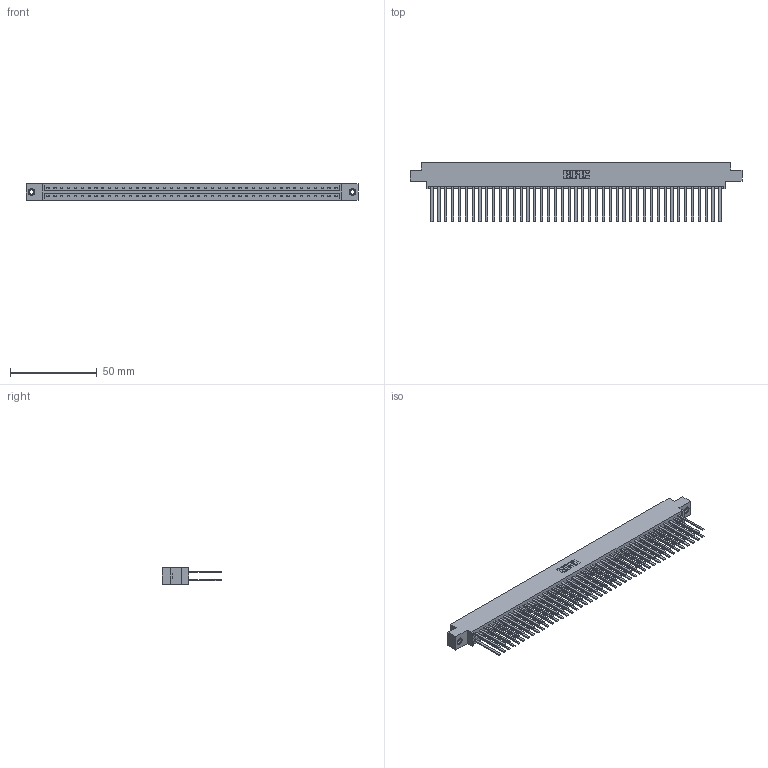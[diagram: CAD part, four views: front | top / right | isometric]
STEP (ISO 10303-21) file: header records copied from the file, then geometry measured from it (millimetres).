
FILE_DESCRIPTION (( 'STEP AP203' ), '1' );
FILE_NAME ('833-086-544-807.STEP', '2020-06-06T03:47:48', ( '' ), ( '' ), 'SwSTEP 2.0', 'SolidWorks 2020', '' );
FILE_SCHEMA (( 'CONFIG_CONTROL_DESIGN' ));
Length unit declared in the file: inch
Products named in the file (4): 345-292-001_345-293-144; 833 Part_Offset - .156 Dia - TI; 833-086-544-807; 345-250-001_345-250-005-103
Assembly tree (89 placements, depth 2):
  833-086-544-807
    833 Part_Offset - .156 Dia - TI
    345-292-001_345-293-144  x86
    345-250-001_345-250-005-103  x2
Bounding box: 191.92 x 34.3 x 9.4 mm (x, y, z)
Volume: 20567.8 mm3; surface area: 28463.5 mm2
Topology: 89 solids, 89 shells, 4134 faces, 12241 edges, 8038 vertices
Faces by surface type: plane 2858, cylinder 1260, cone 12, torus 4
Entity records: 28668 total; most frequent: CARTESIAN_POINT 4733, ORIENTED_EDGE 4662, DIRECTION 4069, EDGE_CURVE 2331, LINE 2187, VECTOR 2187, VERTEX_POINT 1548, AXIS2_PLACEMENT_3D 941
